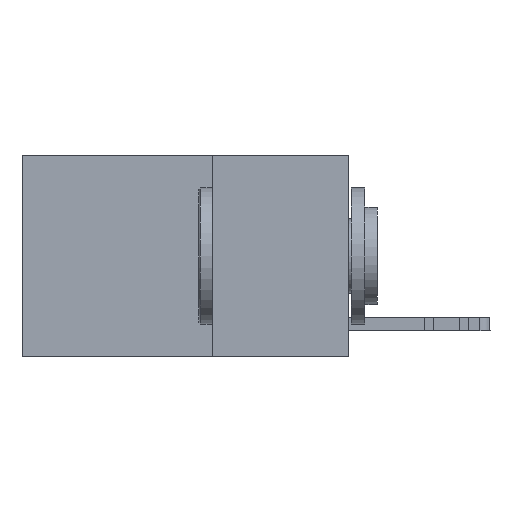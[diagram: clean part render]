
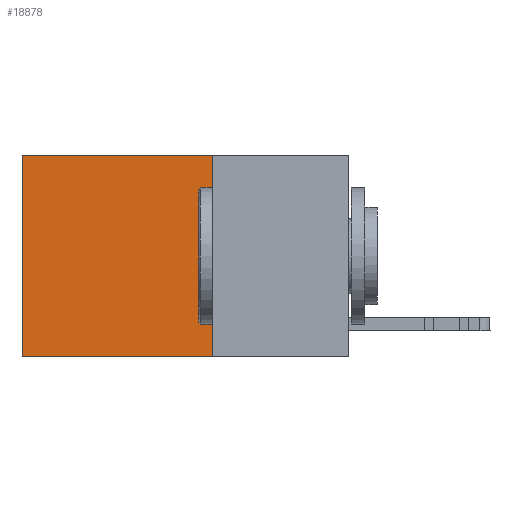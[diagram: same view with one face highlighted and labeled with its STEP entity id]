
A CAD part, left-side view. The second image highlights one B-rep face of the part: STEP entity #18878.
In plain terms, the highlighted planar face has unit normal (-1, 0, 0).
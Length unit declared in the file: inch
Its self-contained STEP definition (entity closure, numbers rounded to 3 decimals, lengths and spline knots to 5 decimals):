
#1799 = CARTESIAN_POINT ( 'NONE',  ( 0.2625, 0.25, 0. ) ) ;
#2444 = VECTOR ( 'NONE', #25823, 39.37008 ) ;
#2897 = CARTESIAN_POINT ( 'NONE',  ( 0.2625, 0.25, 0. ) ) ;
#4094 = EDGE_CURVE ( 'NONE', #9016, #24181, #21045, .T. ) ;
#5171 = EDGE_CURVE ( 'NONE', #15770, #9016, #29069, .T. ) ;
#5389 = DIRECTION ( 'NONE',  ( 0., 1., 0. ) ) ;
#5618 = VECTOR ( 'NONE', #5389, 39.37008 ) ;
#6875 = CARTESIAN_POINT ( 'NONE',  ( 0.2625, 0.6, 0. ) ) ;
#8653 = DIRECTION ( 'NONE',  ( 0., 0., -1. ) ) ;
#9016 = VERTEX_POINT ( 'NONE', #26676 ) ;
#9425 = PLANE ( 'NONE',  #11508 ) ;
#9597 = CARTESIAN_POINT ( 'NONE',  ( 0.2625, 0.25, 0. ) ) ;
#9953 = ORIENTED_EDGE ( 'NONE', *, *, #20056, .F. ) ;
#10625 = VECTOR ( 'NONE', #8653, 39.37008 ) ;
#11508 = AXIS2_PLACEMENT_3D ( 'NONE', #2897, #21103, #23710 ) ;
#12070 = ORIENTED_EDGE ( 'NONE', *, *, #5171, .T. ) ;
#14744 = CARTESIAN_POINT ( 'NONE',  ( 0.2625, 0.6, -0.37 ) ) ;
#14990 = CARTESIAN_POINT ( 'NONE',  ( 0.2625, 0.25, -0.37 ) ) ;
#15770 = VERTEX_POINT ( 'NONE', #9597 ) ;
#16804 = EDGE_LOOP ( 'NONE', ( #19967, #9953, #26853, #12070 ) ) ;
#16947 = VERTEX_POINT ( 'NONE', #14990 ) ;
#18878 = ADVANCED_FACE ( 'NONE', ( #26340 ), #9425, .F. ) ;
#19967 = ORIENTED_EDGE ( 'NONE', *, *, #4094, .T. ) ;
#20056 = EDGE_CURVE ( 'NONE', #16947, #24181, #21738, .T. ) ;
#20192 = LINE ( 'NONE', #1799, #10625 ) ;
#21045 = LINE ( 'NONE', #6875, #2444 ) ;
#21103 = DIRECTION ( 'NONE',  ( 1., 0., 0. ) ) ;
#21738 = LINE ( 'NONE', #21889, #5618 ) ;
#21833 = CARTESIAN_POINT ( 'NONE',  ( 0.2625, 0.25, 0. ) ) ;
#21889 = CARTESIAN_POINT ( 'NONE',  ( 0.2625, 0.25, -0.37 ) ) ;
#23685 = VECTOR ( 'NONE', #28607, 39.37008 ) ;
#23710 = DIRECTION ( 'NONE',  ( 0., 0., -1. ) ) ;
#24181 = VERTEX_POINT ( 'NONE', #14744 ) ;
#25823 = DIRECTION ( 'NONE',  ( 0., 0., -1. ) ) ;
#26340 = FACE_OUTER_BOUND ( 'NONE', #16804, .T. ) ;
#26676 = CARTESIAN_POINT ( 'NONE',  ( 0.2625, 0.6, 0. ) ) ;
#26853 = ORIENTED_EDGE ( 'NONE', *, *, #28539, .F. ) ;
#28539 = EDGE_CURVE ( 'NONE', #15770, #16947, #20192, .T. ) ;
#28607 = DIRECTION ( 'NONE',  ( 0., 1., 0. ) ) ;
#29069 = LINE ( 'NONE', #21833, #23685 ) ;
